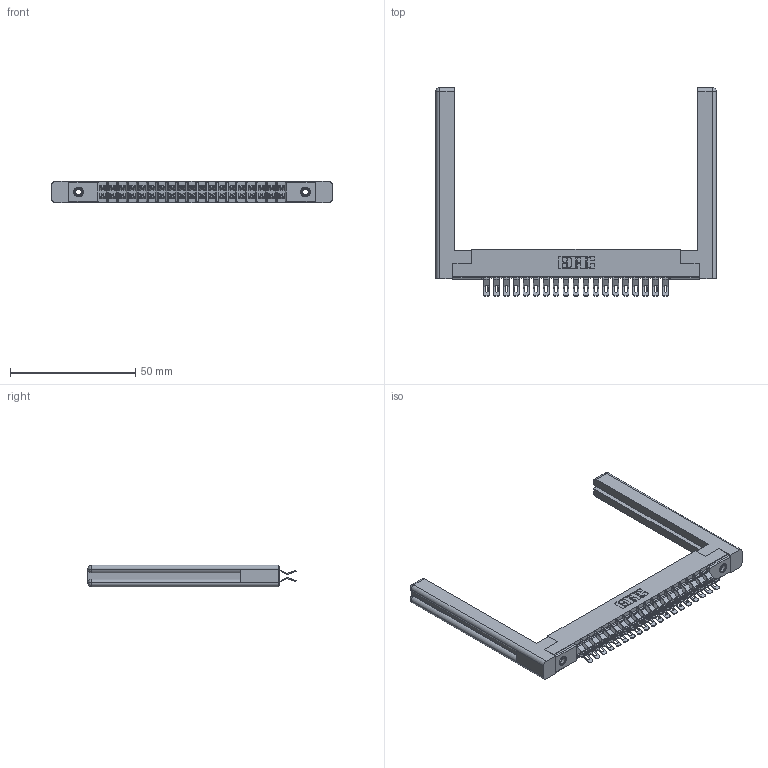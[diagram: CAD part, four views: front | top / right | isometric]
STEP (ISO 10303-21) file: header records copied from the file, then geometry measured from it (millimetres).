
FILE_DESCRIPTION (( 'STEP AP203' ), '1' );
FILE_NAME ('307-038-555-258.STEP', '2019-09-06T04:42:07', ( '' ), ( '' ), 'SwSTEP 2.0', 'SolidWorks 2016', '' );
FILE_SCHEMA (( 'CONFIG_CONTROL_DESIGN' ));
Length unit declared in the file: inch
Products named in the file (5): 307 Part_.156 Dia Mounting Holes; 307-220-058; 307-290-001_555; 345-250-001_345-250-001-102; 307-038-555-258
Assembly tree (43 placements, depth 2):
  307-038-555-258
    307 Part_.156 Dia Mounting Holes
    307-290-001_555  x38
    307-220-058  x2
    345-250-001_345-250-001-102  x2
Bounding box: 111.91 x 83.06 x 8.71 mm (x, y, z)
Volume: 15120.4 mm3; surface area: 18688.3 mm2
Topology: 43 solids, 43 shells, 2598 faces, 7555 edges, 4918 vertices
Faces by surface type: plane 1446, cylinder 1088, sphere 40, torus 12, cone 12
Entity records: 22902 total; most frequent: CARTESIAN_POINT 3778, ORIENTED_EDGE 3686, DIRECTION 3675, EDGE_CURVE 1843, LINE 1389, VECTOR 1389, VERTEX_POINT 1192, AXIS2_PLACEMENT_3D 1143
